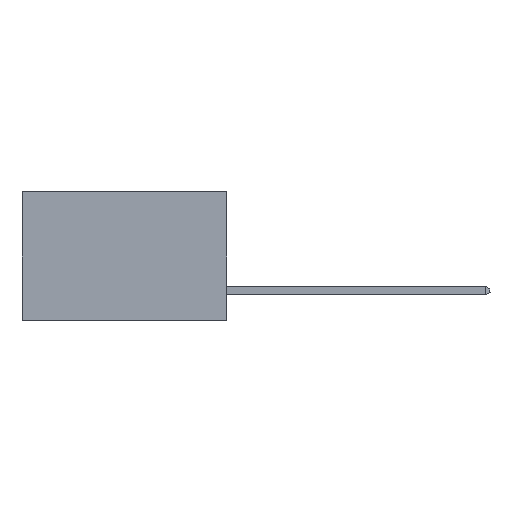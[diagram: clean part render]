
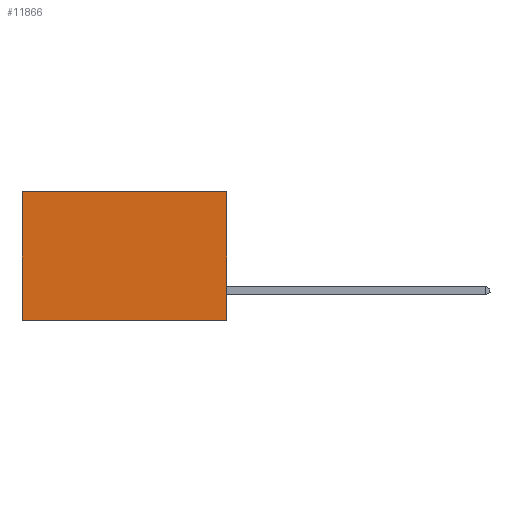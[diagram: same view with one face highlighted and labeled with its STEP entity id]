
A CAD part, left-side view. The second image highlights one B-rep face of the part: STEP entity #11866.
In plain terms, the highlighted planar face has unit normal (-1, 0, 0).
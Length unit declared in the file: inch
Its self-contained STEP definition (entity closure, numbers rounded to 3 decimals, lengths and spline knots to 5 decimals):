
#992 = LINE ( 'NONE', #1412, #1717 ) ;
#1412 = CARTESIAN_POINT ( 'NONE',  ( 0.277, 0.59, -0.37 ) ) ;
#1599 = DIRECTION ( 'NONE',  ( 0., 0., -1. ) ) ;
#1717 = VECTOR ( 'NONE', #1599, 39.37008 ) ;
#4716 = VERTEX_POINT ( 'NONE', #6194 ) ;
#5206 = EDGE_LOOP ( 'NONE', ( #29619, #14307, #10463, #18851 ) ) ;
#5243 = LINE ( 'NONE', #10567, #29615 ) ;
#5614 = CARTESIAN_POINT ( 'NONE',  ( 0.277, 0., 0. ) ) ;
#6194 = CARTESIAN_POINT ( 'NONE',  ( 0.277, 0.59, 0. ) ) ;
#6885 = VERTEX_POINT ( 'NONE', #22105 ) ;
#7908 = EDGE_CURVE ( 'NONE', #4716, #6885, #992, .T. ) ;
#7959 = PLANE ( 'NONE',  #15064 ) ;
#10463 = ORIENTED_EDGE ( 'NONE', *, *, #14851, .F. ) ;
#10466 = EDGE_CURVE ( 'NONE', #18203, #4716, #25778, .T. ) ;
#10567 = CARTESIAN_POINT ( 'NONE',  ( 0.277, 0., -0.37 ) ) ;
#11824 = VERTEX_POINT ( 'NONE', #19704 ) ;
#11866 = ADVANCED_FACE ( 'NONE', ( #27972 ), #7959, .F. ) ;
#12751 = DIRECTION ( 'NONE',  ( 0., 0., -1. ) ) ;
#14307 = ORIENTED_EDGE ( 'NONE', *, *, #19752, .F. ) ;
#14851 = EDGE_CURVE ( 'NONE', #18203, #11824, #5243, .T. ) ;
#15064 = AXIS2_PLACEMENT_3D ( 'NONE', #17390, #26898, #12751 ) ;
#15804 = VECTOR ( 'NONE', #25256, 39.37008 ) ;
#16541 = LINE ( 'NONE', #29889, #15804 ) ;
#16836 = DIRECTION ( 'NONE',  ( 0., 1., 0. ) ) ;
#17005 = CARTESIAN_POINT ( 'NONE',  ( 0.277, 0., 0. ) ) ;
#17390 = CARTESIAN_POINT ( 'NONE',  ( 0.277, 0., -0.37 ) ) ;
#18203 = VERTEX_POINT ( 'NONE', #5614 ) ;
#18851 = ORIENTED_EDGE ( 'NONE', *, *, #10466, .T. ) ;
#19494 = VECTOR ( 'NONE', #16836, 39.37008 ) ;
#19704 = CARTESIAN_POINT ( 'NONE',  ( 0.277, 0., -0.37 ) ) ;
#19752 = EDGE_CURVE ( 'NONE', #11824, #6885, #16541, .T. ) ;
#20025 = DIRECTION ( 'NONE',  ( 0., 0., -1. ) ) ;
#22105 = CARTESIAN_POINT ( 'NONE',  ( 0.277, 0.59, -0.37 ) ) ;
#25256 = DIRECTION ( 'NONE',  ( 0., 1., 0. ) ) ;
#25778 = LINE ( 'NONE', #17005, #19494 ) ;
#26898 = DIRECTION ( 'NONE',  ( 1., 0., 0. ) ) ;
#27972 = FACE_OUTER_BOUND ( 'NONE', #5206, .T. ) ;
#29615 = VECTOR ( 'NONE', #20025, 39.37008 ) ;
#29619 = ORIENTED_EDGE ( 'NONE', *, *, #7908, .T. ) ;
#29889 = CARTESIAN_POINT ( 'NONE',  ( 0.277, 0., -0.37 ) ) ;
